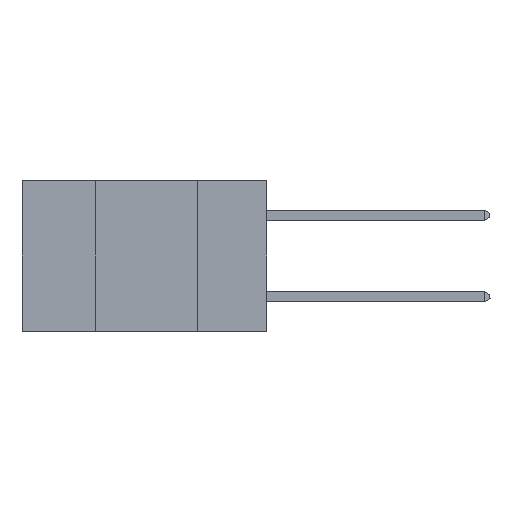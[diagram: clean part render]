
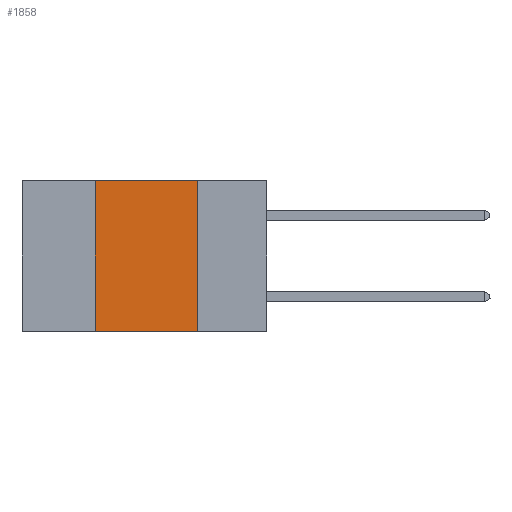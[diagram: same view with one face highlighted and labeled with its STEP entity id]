
A CAD part, left-side view. The second image highlights one B-rep face of the part: STEP entity #1858.
In plain terms, the highlighted planar face has unit normal (-1, 0, 0).
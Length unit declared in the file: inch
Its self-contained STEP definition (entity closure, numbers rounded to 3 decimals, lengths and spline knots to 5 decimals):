
#217 = CARTESIAN_POINT ( 'NONE',  ( 0., 0.6, 0. ) ) ;
#698 = VECTOR ( 'NONE', #2541, 39.37008 ) ;
#724 = CARTESIAN_POINT ( 'NONE',  ( 0., 0.6, 0. ) ) ;
#1347 = FACE_OUTER_BOUND ( 'NONE', #6979, .T. ) ;
#1367 = ORIENTED_EDGE ( 'NONE', *, *, #14335, .F. ) ;
#1538 = AXIS2_PLACEMENT_3D ( 'NONE', #724, #4480, #5495 ) ;
#1646 = CARTESIAN_POINT ( 'NONE',  ( 0., 0.6, -0.37 ) ) ;
#1858 = ADVANCED_FACE ( 'NONE', ( #1347 ), #13888, .F. ) ;
#1993 = DIRECTION ( 'NONE',  ( 0., 0., -1. ) ) ;
#2229 = VERTEX_POINT ( 'NONE', #11541 ) ;
#2541 = DIRECTION ( 'NONE',  ( 0., -1., 0. ) ) ;
#2916 = CARTESIAN_POINT ( 'NONE',  ( 0., 0.42, 0. ) ) ;
#3107 = VERTEX_POINT ( 'NONE', #12867 ) ;
#3872 = LINE ( 'NONE', #217, #698 ) ;
#4117 = DIRECTION ( 'NONE',  ( 0., 0., 1. ) ) ;
#4271 = VECTOR ( 'NONE', #4117, 39.37008 ) ;
#4307 = VECTOR ( 'NONE', #8720, 39.37008 ) ;
#4480 = DIRECTION ( 'NONE',  ( 1., 0., 0. ) ) ;
#4659 = LINE ( 'NONE', #1646, #4307 ) ;
#5305 = LINE ( 'NONE', #13967, #14825 ) ;
#5495 = DIRECTION ( 'NONE',  ( 0., 0., -1. ) ) ;
#5502 = CARTESIAN_POINT ( 'NONE',  ( 0., 0.42, -0.37 ) ) ;
#5563 = ORIENTED_EDGE ( 'NONE', *, *, #15332, .F. ) ;
#5842 = VERTEX_POINT ( 'NONE', #12532 ) ;
#6979 = EDGE_LOOP ( 'NONE', ( #10325, #5563, #1367, #9179 ) ) ;
#8009 = EDGE_CURVE ( 'NONE', #12921, #5842, #4659, .T. ) ;
#8720 = DIRECTION ( 'NONE',  ( 0., -1., 0. ) ) ;
#9179 = ORIENTED_EDGE ( 'NONE', *, *, #8009, .T. ) ;
#10325 = ORIENTED_EDGE ( 'NONE', *, *, #11288, .F. ) ;
#11288 = EDGE_CURVE ( 'NONE', #2229, #5842, #5305, .T. ) ;
#11541 = CARTESIAN_POINT ( 'NONE',  ( 0., 0.17, 0. ) ) ;
#12038 = LINE ( 'NONE', #2916, #4271 ) ;
#12532 = CARTESIAN_POINT ( 'NONE',  ( 0., 0.17, -0.37 ) ) ;
#12867 = CARTESIAN_POINT ( 'NONE',  ( 0., 0.42, 0. ) ) ;
#12921 = VERTEX_POINT ( 'NONE', #5502 ) ;
#13888 = PLANE ( 'NONE',  #1538 ) ;
#13967 = CARTESIAN_POINT ( 'NONE',  ( 0., 0.17, 0. ) ) ;
#14335 = EDGE_CURVE ( 'NONE', #12921, #3107, #12038, .T. ) ;
#14825 = VECTOR ( 'NONE', #1993, 39.37008 ) ;
#15332 = EDGE_CURVE ( 'NONE', #3107, #2229, #3872, .T. ) ;
